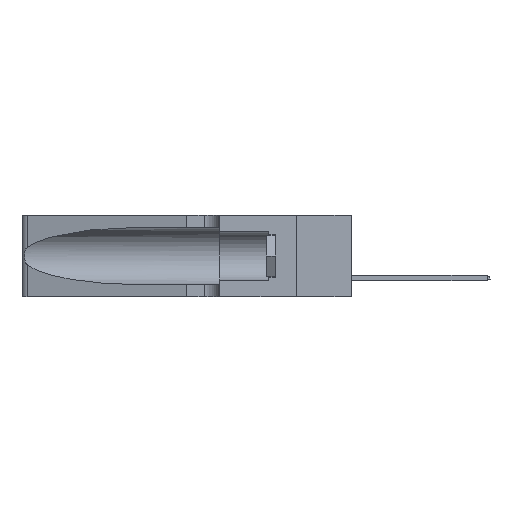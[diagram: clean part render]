
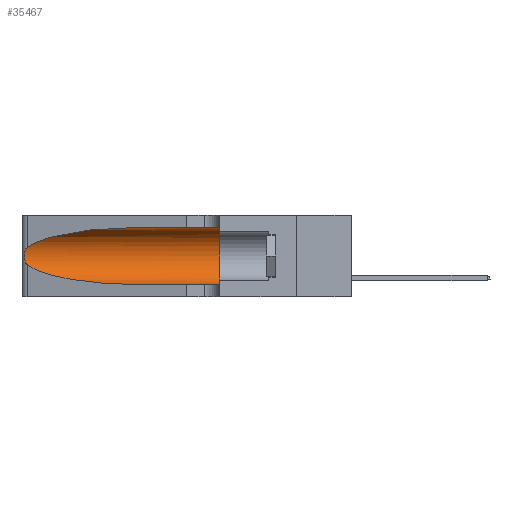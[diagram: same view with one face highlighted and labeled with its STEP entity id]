
A CAD part, left-side view. The second image highlights one B-rep face of the part: STEP entity #35467.
In plain terms, the highlighted cylindrical face has radius 3.308 mm (diameter 6.617 mm), a partial arc.
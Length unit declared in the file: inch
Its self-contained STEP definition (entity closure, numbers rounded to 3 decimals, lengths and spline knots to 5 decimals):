
#314 = ORIENTED_EDGE ( 'NONE', *, *, #4080, .T. ) ;
#609 = CARTESIAN_POINT ( 'NONE',  ( 0.18966, 0.96281, 0.31525 ) ) ;
#1483 = CARTESIAN_POINT ( 'NONE',  ( 0.1305, 1.61858, 0.05475 ) ) ;
#1497 = CARTESIAN_POINT ( 'NONE',  ( 0.26075, 1.23896, 0.19203 ) ) ;
#2754 = B_SPLINE_CURVE_WITH_KNOTS ( 'NONE', 3,
 ( #23887, #9670, #26698, #21172, #31938, #23769, #1497, #12333, #21060, #12717, #10029, #26519, #36212, #27332 ),
 .UNSPECIFIED., .F., .F.,
 ( 4, 2, 2, 2, 2, 2, 4 ),
 ( 0., 0.00027, 0.00053, 0.00107, 0.0016, 0.00187, 0.00214 ),
 .UNSPECIFIED. ) ;
#4080 = EDGE_CURVE ( 'NONE', #6486, #33674, #7010, .T. ) ;
#4971 = CARTESIAN_POINT ( 'NONE',  ( 0.25487, 1.22718, 0.14631 ) ) ;
#5080 = CARTESIAN_POINT ( 'NONE',  ( 0.2373, 1.15595, 0.08982 ) ) ;
#5502 = DIRECTION ( 'NONE',  ( 0., 1., 0. ) ) ;
#5908 = LINE ( 'NONE', #1483, #22539 ) ;
#6486 = VERTEX_POINT ( 'NONE', #32744 ) ;
#7010 =( BOUNDED_CURVE ( )  B_SPLINE_CURVE ( 3, ( #4971, #5080, #7656, #29921 ),
 .UNSPECIFIED., .F., .F. ) 
 B_SPLINE_CURVE_WITH_KNOTS ( ( 4, 4 ),
 ( 3.44316, 4.71239 ),
 .UNSPECIFIED. ) 
 CURVE ( )  GEOMETRIC_REPRESENTATION_ITEM ( )  RATIONAL_B_SPLINE_CURVE ( ( 1., 0.87, 0.87, 1. ) ) 
 REPRESENTATION_ITEM ( '' )  );
#7656 = CARTESIAN_POINT ( 'NONE',  ( 0.18966, 0.96281, 0.05475 ) ) ;
#7737 = VERTEX_POINT ( 'NONE', #20914 ) ;
#8095 = VERTEX_POINT ( 'NONE', #23778 ) ;
#8193 = CARTESIAN_POINT ( 'NONE',  ( 0.1305, 1.61858, 0.185 ) ) ;
#9670 = CARTESIAN_POINT ( 'NONE',  ( 0.25555, 1.22994, 0.2215 ) ) ;
#10029 = CARTESIAN_POINT ( 'NONE',  ( 0.25789, 1.23486, 0.15765 ) ) ;
#11118 = ORIENTED_EDGE ( 'NONE', *, *, #15222, .T. ) ;
#11585 = CARTESIAN_POINT ( 'NONE',  ( 0.2373, 1.15595, 0.28018 ) ) ;
#11639 = ORIENTED_EDGE ( 'NONE', *, *, #18860, .T. ) ;
#12042 = DIRECTION ( 'NONE',  ( 0., -1., 0. ) ) ;
#12053 = ORIENTED_EDGE ( 'NONE', *, *, #12875, .T. ) ;
#12333 = CARTESIAN_POINT ( 'NONE',  ( 0.26075, 1.23896, 0.178 ) ) ;
#12531 = CIRCLE ( 'NONE', #17450, 0.13025 ) ;
#12717 = CARTESIAN_POINT ( 'NONE',  ( 0.25856, 1.23593, 0.16098 ) ) ;
#12875 = EDGE_CURVE ( 'NONE', #33674, #16630, #5908, .T. ) ;
#13762 = DIRECTION ( 'NONE',  ( 0., -1., 0. ) ) ;
#14756 = EDGE_CURVE ( 'NONE', #7737, #8095, #23707, .T. ) ;
#15222 = EDGE_CURVE ( 'NONE', #31689, #6486, #2754, .T. ) ;
#15517 = DIRECTION ( 'NONE',  ( 0., -1., 0. ) ) ;
#16630 = VERTEX_POINT ( 'NONE', #20519 ) ;
#17121 = CARTESIAN_POINT ( 'NONE',  ( 0.1305, 1.61858, 0.31525 ) ) ;
#17450 = AXIS2_PLACEMENT_3D ( 'NONE', #19415, #5502, #30671 ) ;
#18860 = EDGE_CURVE ( 'NONE', #7737, #31689, #19543, .T. ) ;
#19068 = DIRECTION ( 'NONE',  ( 0., 0., -1. ) ) ;
#19415 = CARTESIAN_POINT ( 'NONE',  ( 0.1305, 0.35, 0.185 ) ) ;
#19543 =( BOUNDED_CURVE ( )  B_SPLINE_CURVE ( 3, ( #19927, #609, #11585, #20064 ),
 .UNSPECIFIED., .F., .F. ) 
 B_SPLINE_CURVE_WITH_KNOTS ( ( 4, 4 ),
 ( 1.5708, 2.84003 ),
 .UNSPECIFIED. ) 
 CURVE ( )  GEOMETRIC_REPRESENTATION_ITEM ( )  RATIONAL_B_SPLINE_CURVE ( ( 1., 0.87, 0.87, 1. ) ) 
 REPRESENTATION_ITEM ( '' )  );
#19927 = CARTESIAN_POINT ( 'NONE',  ( 0.1305, 0.72297, 0.31525 ) ) ;
#20064 = CARTESIAN_POINT ( 'NONE',  ( 0.25487, 1.22718, 0.22369 ) ) ;
#20519 = CARTESIAN_POINT ( 'NONE',  ( 0.1305, 0.35, 0.05475 ) ) ;
#20914 = CARTESIAN_POINT ( 'NONE',  ( 0.1305, 0.72297, 0.31525 ) ) ;
#21060 = CARTESIAN_POINT ( 'NONE',  ( 0.26017, 1.23833, 0.17102 ) ) ;
#21172 = CARTESIAN_POINT ( 'NONE',  ( 0.25787, 1.23484, 0.2124 ) ) ;
#21626 = ORIENTED_EDGE ( 'NONE', *, *, #14756, .F. ) ;
#21712 = AXIS2_PLACEMENT_3D ( 'NONE', #8193, #13762, #19068 ) ;
#22539 = VECTOR ( 'NONE', #15517, 39.37008 ) ;
#23707 = LINE ( 'NONE', #17121, #32915 ) ;
#23769 = CARTESIAN_POINT ( 'NONE',  ( 0.26018, 1.23835, 0.19895 ) ) ;
#23778 = CARTESIAN_POINT ( 'NONE',  ( 0.1305, 0.35, 0.31525 ) ) ;
#23887 = CARTESIAN_POINT ( 'NONE',  ( 0.25487, 1.22718, 0.22369 ) ) ;
#24470 = FACE_OUTER_BOUND ( 'NONE', #27820, .T. ) ;
#25598 = EDGE_CURVE ( 'NONE', #8095, #16630, #12531, .T. ) ;
#26175 = CYLINDRICAL_SURFACE ( 'NONE', #21712, 0.13025 ) ;
#26519 = CARTESIAN_POINT ( 'NONE',  ( 0.25639, 1.23186, 0.15144 ) ) ;
#26698 = CARTESIAN_POINT ( 'NONE',  ( 0.25639, 1.23184, 0.21858 ) ) ;
#27332 = CARTESIAN_POINT ( 'NONE',  ( 0.25487, 1.22718, 0.14631 ) ) ;
#27511 = CARTESIAN_POINT ( 'NONE',  ( 0.25487, 1.22718, 0.22369 ) ) ;
#27820 = EDGE_LOOP ( 'NONE', ( #11639, #11118, #314, #12053, #31569, #21626 ) ) ;
#29921 = CARTESIAN_POINT ( 'NONE',  ( 0.1305, 0.72297, 0.05475 ) ) ;
#30671 = DIRECTION ( 'NONE',  ( 0., 0., 1. ) ) ;
#31569 = ORIENTED_EDGE ( 'NONE', *, *, #25598, .F. ) ;
#31689 = VERTEX_POINT ( 'NONE', #27511 ) ;
#31938 = CARTESIAN_POINT ( 'NONE',  ( 0.25854, 1.2359, 0.20912 ) ) ;
#32744 = CARTESIAN_POINT ( 'NONE',  ( 0.25487, 1.22718, 0.14631 ) ) ;
#32915 = VECTOR ( 'NONE', #12042, 39.37008 ) ;
#33674 = VERTEX_POINT ( 'NONE', #35976 ) ;
#35467 = ADVANCED_FACE ( 'NONE', ( #24470 ), #26175, .F. ) ;
#35976 = CARTESIAN_POINT ( 'NONE',  ( 0.1305, 0.72297, 0.05475 ) ) ;
#36212 = CARTESIAN_POINT ( 'NONE',  ( 0.25555, 1.22993, 0.14849 ) ) ;
